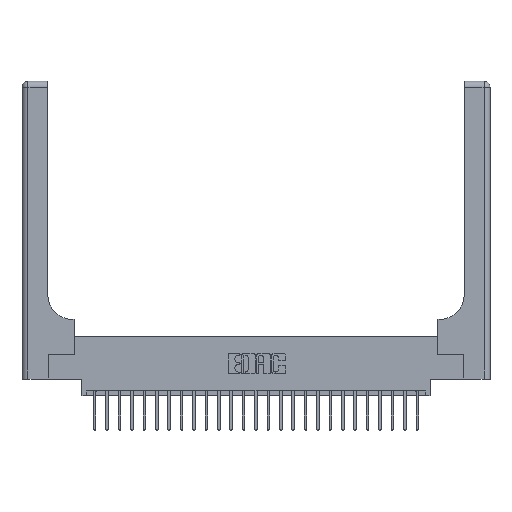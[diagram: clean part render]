
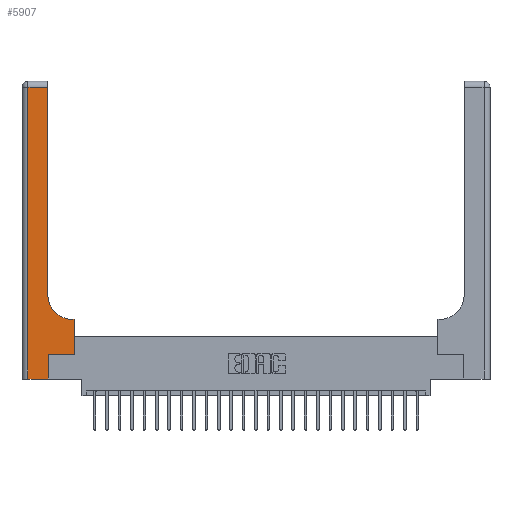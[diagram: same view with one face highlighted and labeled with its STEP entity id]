
A CAD part, top view. The second image highlights one B-rep face of the part: STEP entity #5907.
In plain terms, the highlighted planar face has unit normal (0, 0, 1).
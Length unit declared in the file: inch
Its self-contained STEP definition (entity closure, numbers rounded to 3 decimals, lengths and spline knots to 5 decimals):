
#167 = CARTESIAN_POINT ( 'NONE',  ( 0.06, 3., 0.37 ) ) ;
#512 = VECTOR ( 'NONE', #19804, 39.37008 ) ;
#1798 = VECTOR ( 'NONE', #13391, 39.37008 ) ;
#1883 = EDGE_CURVE ( 'NONE', #13692, #7420, #21477, .T. ) ;
#2829 = VERTEX_POINT ( 'NONE', #10057 ) ;
#3051 = VECTOR ( 'NONE', #23771, 39.37008 ) ;
#3169 = DIRECTION ( 'NONE',  ( 1., 0., 0. ) ) ;
#3226 = CARTESIAN_POINT ( 'NONE',  ( 0.26, 2.94, 0.37 ) ) ;
#3428 = LINE ( 'NONE', #24932, #17494 ) ;
#3480 = AXIS2_PLACEMENT_3D ( 'NONE', #4386, #4509, #20463 ) ;
#3750 = ORIENTED_EDGE ( 'NONE', *, *, #17500, .T. ) ;
#4386 = CARTESIAN_POINT ( 'NONE',  ( 0., 3., 0.37 ) ) ;
#4509 = DIRECTION ( 'NONE',  ( 0., 0., -1. ) ) ;
#5279 = CARTESIAN_POINT ( 'NONE',  ( 0.528, 0.25, 0.37 ) ) ;
#5606 = ORIENTED_EDGE ( 'NONE', *, *, #1883, .T. ) ;
#5907 = ADVANCED_FACE ( 'NONE', ( #22007 ), #15980, .F. ) ;
#6425 = EDGE_CURVE ( 'NONE', #16373, #13692, #3428, .T. ) ;
#6485 = ORIENTED_EDGE ( 'NONE', *, *, #23669, .T. ) ;
#6518 = CARTESIAN_POINT ( 'NONE',  ( 0.26, 0.85, 0.37 ) ) ;
#7420 = VERTEX_POINT ( 'NONE', #23042 ) ;
#8135 = EDGE_CURVE ( 'NONE', #2829, #17912, #24075, .T. ) ;
#8460 = AXIS2_PLACEMENT_3D ( 'NONE', #23154, #19547, #21100 ) ;
#8463 = LINE ( 'NONE', #8704, #12583 ) ;
#8587 = DIRECTION ( 'NONE',  ( 0., 1., 0. ) ) ;
#8704 = CARTESIAN_POINT ( 'NONE',  ( 0.265, 0., 0.37 ) ) ;
#8725 = DIRECTION ( 'NONE',  ( 0., -1., 0. ) ) ;
#9318 = VERTEX_POINT ( 'NONE', #24988 ) ;
#9329 = CARTESIAN_POINT ( 'NONE',  ( 0.26, 0.6, 0.37 ) ) ;
#10057 = CARTESIAN_POINT ( 'NONE',  ( 0.51, 0.6, 0.37 ) ) ;
#10200 = ORIENTED_EDGE ( 'NONE', *, *, #8135, .T. ) ;
#10774 = VERTEX_POINT ( 'NONE', #16963 ) ;
#11469 = ORIENTED_EDGE ( 'NONE', *, *, #12442, .T. ) ;
#11500 = VERTEX_POINT ( 'NONE', #3226 ) ;
#11988 = LINE ( 'NONE', #167, #14559 ) ;
#12442 = EDGE_CURVE ( 'NONE', #17912, #11500, #15146, .T. ) ;
#12583 = VECTOR ( 'NONE', #8587, 39.37008 ) ;
#12940 = DIRECTION ( 'NONE',  ( -1., 0., 0. ) ) ;
#13327 = CARTESIAN_POINT ( 'NONE',  ( 0.26, 3., 0.37 ) ) ;
#13373 = CARTESIAN_POINT ( 'NONE',  ( 0.265, 0.25, 0.37 ) ) ;
#13391 = DIRECTION ( 'NONE',  ( 0., 1., 0. ) ) ;
#13472 = EDGE_CURVE ( 'NONE', #11500, #25055, #15669, .T. ) ;
#13692 = VERTEX_POINT ( 'NONE', #20146 ) ;
#14559 = VECTOR ( 'NONE', #8725, 39.37008 ) ;
#15146 = LINE ( 'NONE', #13327, #19504 ) ;
#15581 = CARTESIAN_POINT ( 'NONE',  ( 0., 0., 0.37 ) ) ;
#15623 = EDGE_LOOP ( 'NONE', ( #11469, #23834, #3750, #18225, #24477, #22183, #5606, #6485, #10200 ) ) ;
#15669 = LINE ( 'NONE', #23887, #3051 ) ;
#15850 = EDGE_CURVE ( 'NONE', #10774, #9318, #21232, .T. ) ;
#15980 = PLANE ( 'NONE',  #3480 ) ;
#16373 = VERTEX_POINT ( 'NONE', #13373 ) ;
#16963 = CARTESIAN_POINT ( 'NONE',  ( 0.06, 0., 0.37 ) ) ;
#17494 = VECTOR ( 'NONE', #3169, 39.37008 ) ;
#17500 = EDGE_CURVE ( 'NONE', #25055, #10774, #11988, .T. ) ;
#17912 = VERTEX_POINT ( 'NONE', #6518 ) ;
#18225 = ORIENTED_EDGE ( 'NONE', *, *, #15850, .T. ) ;
#18738 = CARTESIAN_POINT ( 'NONE',  ( 0.06, 2.94, 0.37 ) ) ;
#18982 = DIRECTION ( 'NONE',  ( 0., 1., 0. ) ) ;
#19504 = VECTOR ( 'NONE', #18982, 39.37008 ) ;
#19547 = DIRECTION ( 'NONE',  ( 0., 0., -1. ) ) ;
#19612 = VECTOR ( 'NONE', #12940, 39.37008 ) ;
#19804 = DIRECTION ( 'NONE',  ( 1., 0., 0. ) ) ;
#20146 = CARTESIAN_POINT ( 'NONE',  ( 0.528, 0.25, 0.37 ) ) ;
#20463 = DIRECTION ( 'NONE',  ( -1., 0., 0. ) ) ;
#21100 = DIRECTION ( 'NONE',  ( 1., 0., 0. ) ) ;
#21232 = LINE ( 'NONE', #15581, #512 ) ;
#21477 = LINE ( 'NONE', #5279, #1798 ) ;
#21779 = EDGE_CURVE ( 'NONE', #9318, #16373, #8463, .T. ) ;
#22007 = FACE_OUTER_BOUND ( 'NONE', #15623, .T. ) ;
#22183 = ORIENTED_EDGE ( 'NONE', *, *, #6425, .T. ) ;
#23042 = CARTESIAN_POINT ( 'NONE',  ( 0.528, 0.6, 0.37 ) ) ;
#23154 = CARTESIAN_POINT ( 'NONE',  ( 0.51, 0.85, 0.37 ) ) ;
#23669 = EDGE_CURVE ( 'NONE', #7420, #2829, #24785, .T. ) ;
#23771 = DIRECTION ( 'NONE',  ( -1., 0., 0. ) ) ;
#23834 = ORIENTED_EDGE ( 'NONE', *, *, #13472, .T. ) ;
#23887 = CARTESIAN_POINT ( 'NONE',  ( 0., 2.94, 0.37 ) ) ;
#24075 = CIRCLE ( 'NONE', #8460, 0.25 ) ;
#24477 = ORIENTED_EDGE ( 'NONE', *, *, #21779, .T. ) ;
#24785 = LINE ( 'NONE', #9329, #19612 ) ;
#24932 = CARTESIAN_POINT ( 'NONE',  ( 0.265, 0.25, 0.37 ) ) ;
#24988 = CARTESIAN_POINT ( 'NONE',  ( 0.265, 0., 0.37 ) ) ;
#25055 = VERTEX_POINT ( 'NONE', #18738 ) ;
